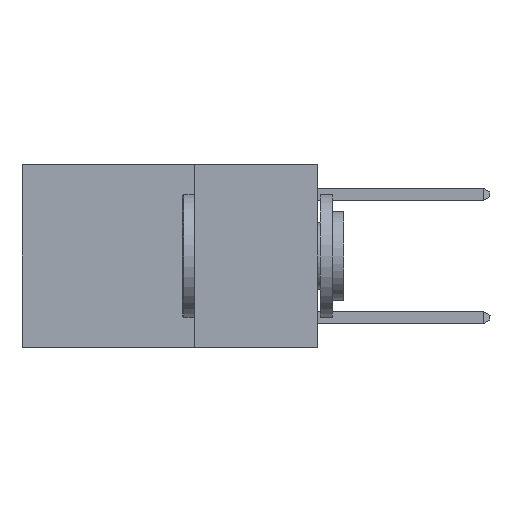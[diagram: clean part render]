
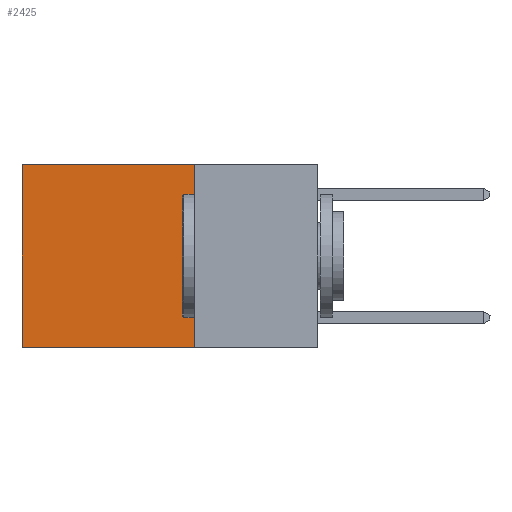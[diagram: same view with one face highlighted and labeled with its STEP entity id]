
A CAD part, left-side view. The second image highlights one B-rep face of the part: STEP entity #2425.
In plain terms, the highlighted planar face has unit normal (-1, 0, 0).
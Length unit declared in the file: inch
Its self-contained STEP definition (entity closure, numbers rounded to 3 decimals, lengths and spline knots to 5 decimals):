
#187 = EDGE_CURVE ( 'NONE', #13152, #11999, #8825, .T. ) ;
#383 = DIRECTION ( 'NONE',  ( 0., 1., 0. ) ) ;
#2425 = ADVANCED_FACE ( 'NONE', ( #19684 ), #22015, .F. ) ;
#4333 = CARTESIAN_POINT ( 'NONE',  ( 0.2625, 0.25, -0.37 ) ) ;
#4745 = CARTESIAN_POINT ( 'NONE',  ( 0.2625, 0.6, 0. ) ) ;
#6420 = ORIENTED_EDGE ( 'NONE', *, *, #19367, .F. ) ;
#7529 = DIRECTION ( 'NONE',  ( 0., 1., 0. ) ) ;
#7716 = CARTESIAN_POINT ( 'NONE',  ( 0.2625, 0.25, 0. ) ) ;
#8107 = LINE ( 'NONE', #4745, #22162 ) ;
#8825 = LINE ( 'NONE', #21822, #13939 ) ;
#9343 = CARTESIAN_POINT ( 'NONE',  ( 0.2625, 0.25, 0. ) ) ;
#9636 = DIRECTION ( 'NONE',  ( 1., 0., 0. ) ) ;
#11999 = VERTEX_POINT ( 'NONE', #4333 ) ;
#12167 = ORIENTED_EDGE ( 'NONE', *, *, #15030, .T. ) ;
#12475 = EDGE_LOOP ( 'NONE', ( #16775, #6420, #20332, #12167 ) ) ;
#12781 = VERTEX_POINT ( 'NONE', #22426 ) ;
#13152 = VERTEX_POINT ( 'NONE', #15861 ) ;
#13939 = VECTOR ( 'NONE', #20291, 39.37008 ) ;
#14446 = EDGE_CURVE ( 'NONE', #12781, #21685, #8107, .T. ) ;
#15030 = EDGE_CURVE ( 'NONE', #13152, #12781, #18510, .T. ) ;
#15786 = DIRECTION ( 'NONE',  ( 0., 0., -1. ) ) ;
#15861 = CARTESIAN_POINT ( 'NONE',  ( 0.2625, 0.25, 0. ) ) ;
#16775 = ORIENTED_EDGE ( 'NONE', *, *, #14446, .T. ) ;
#17492 = VECTOR ( 'NONE', #7529, 39.37008 ) ;
#18076 = CARTESIAN_POINT ( 'NONE',  ( 0.2625, 0.25, -0.37 ) ) ;
#18510 = LINE ( 'NONE', #9343, #22137 ) ;
#18977 = AXIS2_PLACEMENT_3D ( 'NONE', #7716, #9636, #20274 ) ;
#19367 = EDGE_CURVE ( 'NONE', #11999, #21685, #22252, .T. ) ;
#19684 = FACE_OUTER_BOUND ( 'NONE', #12475, .T. ) ;
#20274 = DIRECTION ( 'NONE',  ( 0., 0., -1. ) ) ;
#20291 = DIRECTION ( 'NONE',  ( 0., 0., -1. ) ) ;
#20332 = ORIENTED_EDGE ( 'NONE', *, *, #187, .F. ) ;
#21074 = CARTESIAN_POINT ( 'NONE',  ( 0.2625, 0.6, -0.37 ) ) ;
#21685 = VERTEX_POINT ( 'NONE', #21074 ) ;
#21822 = CARTESIAN_POINT ( 'NONE',  ( 0.2625, 0.25, 0. ) ) ;
#22015 = PLANE ( 'NONE',  #18977 ) ;
#22137 = VECTOR ( 'NONE', #383, 39.37008 ) ;
#22162 = VECTOR ( 'NONE', #15786, 39.37008 ) ;
#22252 = LINE ( 'NONE', #18076, #17492 ) ;
#22426 = CARTESIAN_POINT ( 'NONE',  ( 0.2625, 0.6, 0. ) ) ;
